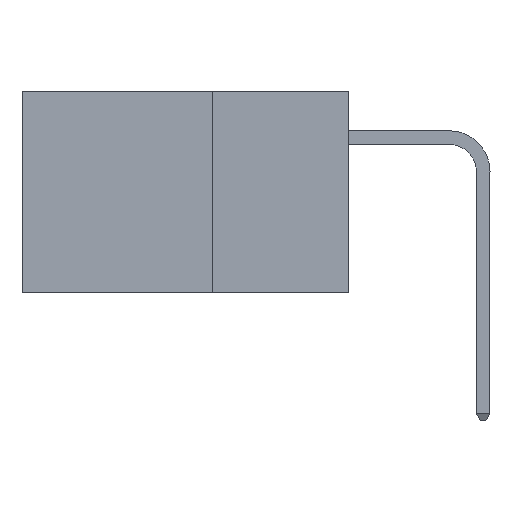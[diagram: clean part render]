
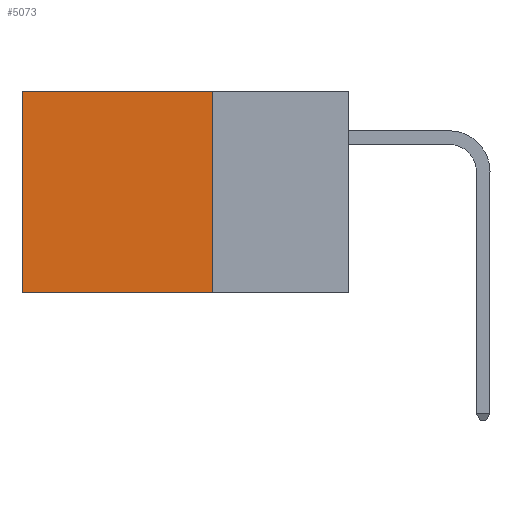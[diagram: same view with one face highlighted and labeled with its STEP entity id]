
A CAD part, left-side view. The second image highlights one B-rep face of the part: STEP entity #5073.
In plain terms, the highlighted planar face has unit normal (-1, 0, 0).
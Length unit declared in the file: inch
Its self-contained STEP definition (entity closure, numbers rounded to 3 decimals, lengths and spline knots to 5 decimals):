
#252 = DIRECTION ( 'NONE',  ( 0., 0., -1. ) ) ;
#2568 = DIRECTION ( 'NONE',  ( 1., 0., 0. ) ) ;
#3481 = VERTEX_POINT ( 'NONE', #24397 ) ;
#3600 = ORIENTED_EDGE ( 'NONE', *, *, #29533, .T. ) ;
#4686 = EDGE_CURVE ( 'NONE', #9019, #3481, #19436, .T. ) ;
#5073 = ADVANCED_FACE ( 'NONE', ( #31036 ), #28895, .F. ) ;
#5909 = ORIENTED_EDGE ( 'NONE', *, *, #4686, .F. ) ;
#6071 = CARTESIAN_POINT ( 'NONE',  ( 0.2875, 0.6, 0. ) ) ;
#6159 = ORIENTED_EDGE ( 'NONE', *, *, #11950, .F. ) ;
#6390 = EDGE_LOOP ( 'NONE', ( #3600, #6159, #5909, #27181 ) ) ;
#6833 = LINE ( 'NONE', #24639, #23673 ) ;
#8098 = VECTOR ( 'NONE', #13303, 39.37008 ) ;
#9019 = VERTEX_POINT ( 'NONE', #29298 ) ;
#9141 = DIRECTION ( 'NONE',  ( 0., 0., -1. ) ) ;
#9214 = VERTEX_POINT ( 'NONE', #18483 ) ;
#10161 = CARTESIAN_POINT ( 'NONE',  ( 0.2875, 0.25, 0. ) ) ;
#11950 = EDGE_CURVE ( 'NONE', #3481, #23592, #14483, .T. ) ;
#12604 = AXIS2_PLACEMENT_3D ( 'NONE', #14633, #2568, #252 ) ;
#13303 = DIRECTION ( 'NONE',  ( 0., 1., 0. ) ) ;
#14483 = LINE ( 'NONE', #25143, #8098 ) ;
#14633 = CARTESIAN_POINT ( 'NONE',  ( 0.2875, 0.25, 0. ) ) ;
#15091 = EDGE_CURVE ( 'NONE', #9019, #9214, #6833, .T. ) ;
#15256 = VECTOR ( 'NONE', #9141, 39.37008 ) ;
#18483 = CARTESIAN_POINT ( 'NONE',  ( 0.2875, 0.6, 0. ) ) ;
#19436 = LINE ( 'NONE', #10161, #25059 ) ;
#22585 = DIRECTION ( 'NONE',  ( 0., 0., -1. ) ) ;
#23592 = VERTEX_POINT ( 'NONE', #27201 ) ;
#23673 = VECTOR ( 'NONE', #24530, 39.37008 ) ;
#24397 = CARTESIAN_POINT ( 'NONE',  ( 0.2875, 0.25, -0.37 ) ) ;
#24530 = DIRECTION ( 'NONE',  ( 0., 1., 0. ) ) ;
#24639 = CARTESIAN_POINT ( 'NONE',  ( 0.2875, 0.25, 0. ) ) ;
#25059 = VECTOR ( 'NONE', #22585, 39.37008 ) ;
#25143 = CARTESIAN_POINT ( 'NONE',  ( 0.2875, 0.25, -0.37 ) ) ;
#26500 = LINE ( 'NONE', #6071, #15256 ) ;
#27181 = ORIENTED_EDGE ( 'NONE', *, *, #15091, .T. ) ;
#27201 = CARTESIAN_POINT ( 'NONE',  ( 0.2875, 0.6, -0.37 ) ) ;
#28895 = PLANE ( 'NONE',  #12604 ) ;
#29298 = CARTESIAN_POINT ( 'NONE',  ( 0.2875, 0.25, 0. ) ) ;
#29533 = EDGE_CURVE ( 'NONE', #9214, #23592, #26500, .T. ) ;
#31036 = FACE_OUTER_BOUND ( 'NONE', #6390, .T. ) ;
